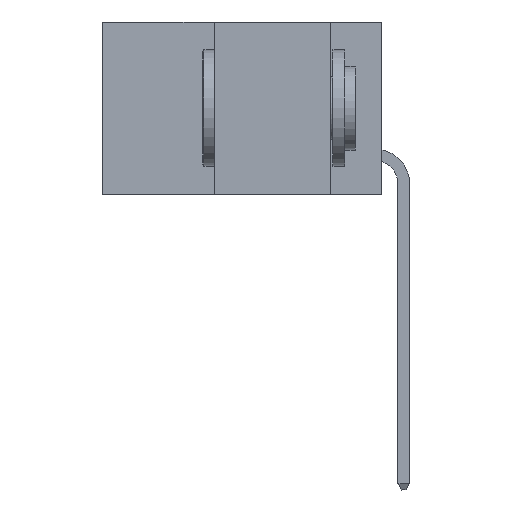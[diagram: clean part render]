
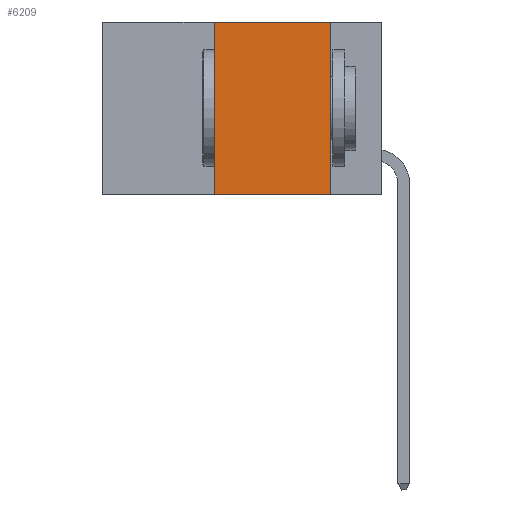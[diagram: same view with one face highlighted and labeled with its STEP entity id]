
A CAD part, left-side view. The second image highlights one B-rep face of the part: STEP entity #6209.
In plain terms, the highlighted planar face has unit normal (-1, 0, 0).
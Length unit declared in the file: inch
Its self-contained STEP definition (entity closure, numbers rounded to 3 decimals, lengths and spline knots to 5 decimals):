
#614 = FACE_OUTER_BOUND ( 'NONE', #1657, .T. ) ;
#1657 = EDGE_LOOP ( 'NONE', ( #6057, #6106, #6890, #10551 ) ) ;
#2045 = CARTESIAN_POINT ( 'NONE',  ( 0., 0.6, 0. ) ) ;
#2491 = LINE ( 'NONE', #14862, #12615 ) ;
#3594 = AXIS2_PLACEMENT_3D ( 'NONE', #4999, #6291, #14951 ) ;
#4464 = CARTESIAN_POINT ( 'NONE',  ( 0., 0.11, -0.37 ) ) ;
#4682 = VERTEX_POINT ( 'NONE', #4464 ) ;
#4999 = CARTESIAN_POINT ( 'NONE',  ( 0., 0.6, 0. ) ) ;
#6057 = ORIENTED_EDGE ( 'NONE', *, *, #10458, .F. ) ;
#6106 = ORIENTED_EDGE ( 'NONE', *, *, #12490, .F. ) ;
#6118 = LINE ( 'NONE', #10488, #9140 ) ;
#6160 = CARTESIAN_POINT ( 'NONE',  ( 0., 0.36, 0. ) ) ;
#6209 = ADVANCED_FACE ( 'NONE', ( #614 ), #11305, .F. ) ;
#6291 = DIRECTION ( 'NONE',  ( 1., 0., 0. ) ) ;
#6890 = ORIENTED_EDGE ( 'NONE', *, *, #14787, .F. ) ;
#7338 = DIRECTION ( 'NONE',  ( 0., -1., 0. ) ) ;
#7771 = VERTEX_POINT ( 'NONE', #12928 ) ;
#8751 = DIRECTION ( 'NONE',  ( 0., -1., 0. ) ) ;
#9140 = VECTOR ( 'NONE', #9233, 39.37008 ) ;
#9233 = DIRECTION ( 'NONE',  ( 0., 0., -1. ) ) ;
#10458 = EDGE_CURVE ( 'NONE', #7771, #4682, #6118, .T. ) ;
#10488 = CARTESIAN_POINT ( 'NONE',  ( 0., 0.11, 0. ) ) ;
#10551 = ORIENTED_EDGE ( 'NONE', *, *, #12552, .T. ) ;
#10995 = LINE ( 'NONE', #2045, #14197 ) ;
#11170 = CARTESIAN_POINT ( 'NONE',  ( 0., 0.6, -0.37 ) ) ;
#11305 = PLANE ( 'NONE',  #3594 ) ;
#12413 = DIRECTION ( 'NONE',  ( 0., 0., 1. ) ) ;
#12490 = EDGE_CURVE ( 'NONE', #14099, #7771, #10995, .T. ) ;
#12552 = EDGE_CURVE ( 'NONE', #15667, #4682, #13443, .T. ) ;
#12615 = VECTOR ( 'NONE', #12413, 39.37008 ) ;
#12928 = CARTESIAN_POINT ( 'NONE',  ( 0., 0.11, 0. ) ) ;
#13045 = VECTOR ( 'NONE', #8751, 39.37008 ) ;
#13137 = CARTESIAN_POINT ( 'NONE',  ( 0., 0.36, -0.37 ) ) ;
#13443 = LINE ( 'NONE', #11170, #13045 ) ;
#14099 = VERTEX_POINT ( 'NONE', #6160 ) ;
#14197 = VECTOR ( 'NONE', #7338, 39.37008 ) ;
#14787 = EDGE_CURVE ( 'NONE', #15667, #14099, #2491, .T. ) ;
#14862 = CARTESIAN_POINT ( 'NONE',  ( 0., 0.36, 0. ) ) ;
#14951 = DIRECTION ( 'NONE',  ( 0., 0., -1. ) ) ;
#15667 = VERTEX_POINT ( 'NONE', #13137 ) ;
